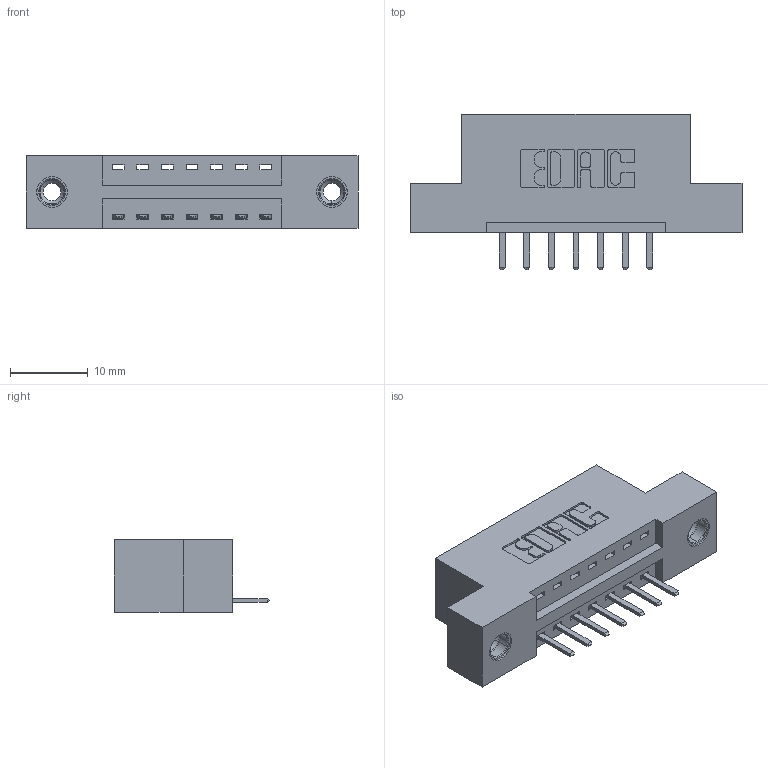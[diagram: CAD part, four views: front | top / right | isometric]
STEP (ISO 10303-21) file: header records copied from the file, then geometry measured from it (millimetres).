
FILE_DESCRIPTION (( 'STEP AP203' ), '1' );
FILE_NAME ('396-007-520-108.STEP', '2018-08-30T23:25:58', ( '' ), ( '' ), 'SwSTEP 2.0', 'SolidWorks 2016', '' );
FILE_SCHEMA (( 'CONFIG_CONTROL_DESIGN' ));
Length unit declared in the file: inch
Products named in the file (4): 345-292-001_345-293-120; 345-250-001_345-250-003-102; 396-007-520-108; 346 Part_Flush Mounting Lugs - 0.156 Dia-TI
Assembly tree (10 placements, depth 2):
  396-007-520-108
    346 Part_Flush Mounting Lugs - 0.156 Dia-TI
    345-292-001_345-293-120  x7
    345-250-001_345-250-003-102  x2
Bounding box: 42.8 x 20.02 x 9.4 mm (x, y, z)
Volume: 3829 mm3; surface area: 4362.7 mm2
Topology: 10 solids, 10 shells, 616 faces, 1753 edges, 1142 vertices
Faces by surface type: plane 402, cylinder 198, cone 12, torus 4
Entity records: 10356 total; most frequent: CARTESIAN_POINT 1780, ORIENTED_EDGE 1702, DIRECTION 1627, EDGE_CURVE 851, LINE 667, VECTOR 667, VERTEX_POINT 560, AXIS2_PLACEMENT_3D 480
